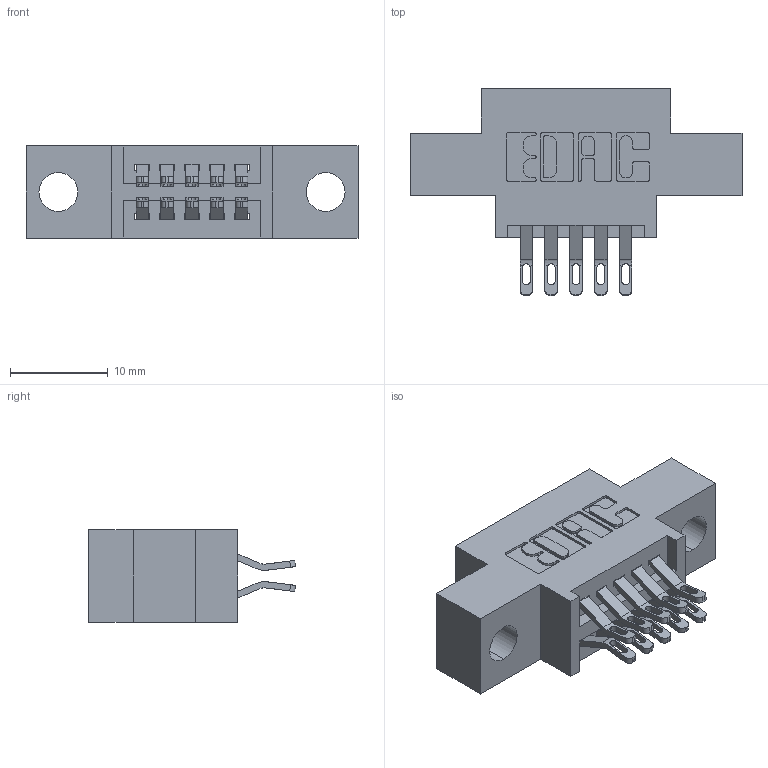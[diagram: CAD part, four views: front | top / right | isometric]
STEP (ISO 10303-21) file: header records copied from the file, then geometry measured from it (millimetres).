
FILE_DESCRIPTION (( 'STEP AP203' ), '1' );
FILE_NAME ('345-010-555-804.STEP', '2021-05-19T15:32:22', ( '' ), ( '' ), 'SwSTEP 2.0', 'SolidWorks 2020', '' );
FILE_SCHEMA (( 'CONFIG_CONTROL_DESIGN' ));
Length unit declared in the file: inch
Products named in the file (3): 345-010-555-804; 345 Part_0.170 Offset - 0.156 Dia-TI; 345-292-001_555 Tail
Assembly tree (11 placements, depth 2):
  345-010-555-804
    345 Part_0.170 Offset - 0.156 Dia-TI
    345-292-001_555 Tail  x10
Bounding box: 33.91 x 21.13 x 9.4 mm (x, y, z)
Volume: 2760.2 mm3; surface area: 3459.3 mm2
Topology: 11 solids, 11 shells, 704 faces, 2159 edges, 1438 vertices
Faces by surface type: plane 408, cylinder 296
Entity records: 9781 total; most frequent: CARTESIAN_POINT 1716, ORIENTED_EDGE 1618, DIRECTION 1525, EDGE_CURVE 809, LINE 637, VECTOR 637, VERTEX_POINT 538, AXIS2_PLACEMENT_3D 444
